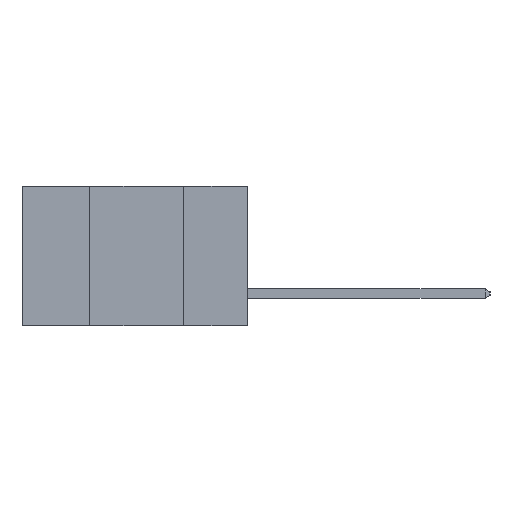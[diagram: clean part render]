
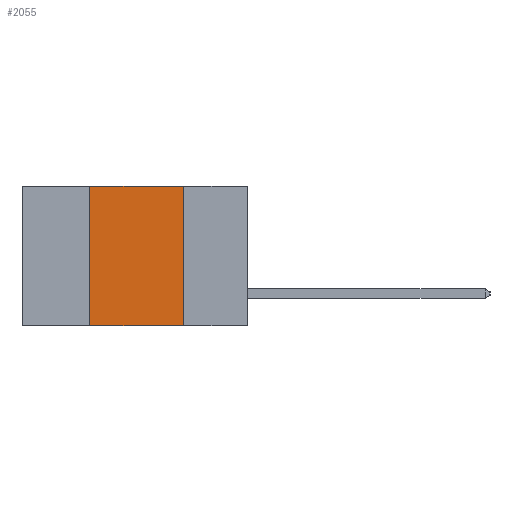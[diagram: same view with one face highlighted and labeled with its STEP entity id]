
A CAD part, left-side view. The second image highlights one B-rep face of the part: STEP entity #2055.
In plain terms, the highlighted planar face has unit normal (-1, 0, 0).
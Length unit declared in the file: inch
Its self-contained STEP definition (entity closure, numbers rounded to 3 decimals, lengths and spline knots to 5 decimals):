
#391 = VERTEX_POINT ( 'NONE', #6027 ) ;
#1665 = CARTESIAN_POINT ( 'NONE',  ( 0., 0.17, -0.37 ) ) ;
#1932 = CARTESIAN_POINT ( 'NONE',  ( 0., 0.17, -0.37 ) ) ;
#2007 = VERTEX_POINT ( 'NONE', #8276 ) ;
#2055 = ADVANCED_FACE ( 'NONE', ( #8479 ), #3976, .F. ) ;
#2655 = CARTESIAN_POINT ( 'NONE',  ( 0., 0.6, 0. ) ) ;
#2807 = VECTOR ( 'NONE', #7940, 39.37008 ) ;
#3788 = AXIS2_PLACEMENT_3D ( 'NONE', #2655, #3861, #4681 ) ;
#3816 = VERTEX_POINT ( 'NONE', #7583 ) ;
#3861 = DIRECTION ( 'NONE',  ( 1., 0., 0. ) ) ;
#3976 = PLANE ( 'NONE',  #3788 ) ;
#4073 = VECTOR ( 'NONE', #4598, 39.37008 ) ;
#4598 = DIRECTION ( 'NONE',  ( 0., -1., 0. ) ) ;
#4655 = CARTESIAN_POINT ( 'NONE',  ( 0., 0.6, 0. ) ) ;
#4681 = DIRECTION ( 'NONE',  ( 0., 0., -1. ) ) ;
#5644 = DIRECTION ( 'NONE',  ( 0., 0., -1. ) ) ;
#6027 = CARTESIAN_POINT ( 'NONE',  ( 0., 0.42, 0. ) ) ;
#6118 = LINE ( 'NONE', #4655, #4073 ) ;
#6130 = DIRECTION ( 'NONE',  ( 0., -1., 0. ) ) ;
#6424 = CARTESIAN_POINT ( 'NONE',  ( 0., 0.6, -0.37 ) ) ;
#6663 = EDGE_CURVE ( 'NONE', #3816, #9134, #8520, .T. ) ;
#6905 = LINE ( 'NONE', #8076, #2807 ) ;
#7148 = EDGE_CURVE ( 'NONE', #3816, #391, #6905, .T. ) ;
#7583 = CARTESIAN_POINT ( 'NONE',  ( 0., 0.42, -0.37 ) ) ;
#7614 = ORIENTED_EDGE ( 'NONE', *, *, #6663, .T. ) ;
#7630 = ORIENTED_EDGE ( 'NONE', *, *, #7148, .F. ) ;
#7653 = EDGE_CURVE ( 'NONE', #391, #2007, #6118, .T. ) ;
#7687 = ORIENTED_EDGE ( 'NONE', *, *, #7653, .F. ) ;
#7940 = DIRECTION ( 'NONE',  ( 0., 0., 1. ) ) ;
#7990 = ORIENTED_EDGE ( 'NONE', *, *, #9550, .F. ) ;
#8076 = CARTESIAN_POINT ( 'NONE',  ( 0., 0.42, -0.37 ) ) ;
#8276 = CARTESIAN_POINT ( 'NONE',  ( 0., 0.17, 0. ) ) ;
#8479 = FACE_OUTER_BOUND ( 'NONE', #9296, .T. ) ;
#8520 = LINE ( 'NONE', #6424, #9918 ) ;
#9040 = VECTOR ( 'NONE', #5644, 39.37008 ) ;
#9134 = VERTEX_POINT ( 'NONE', #1932 ) ;
#9251 = LINE ( 'NONE', #1665, #9040 ) ;
#9296 = EDGE_LOOP ( 'NONE', ( #7990, #7687, #7630, #7614 ) ) ;
#9550 = EDGE_CURVE ( 'NONE', #2007, #9134, #9251, .T. ) ;
#9918 = VECTOR ( 'NONE', #6130, 39.37008 ) ;
